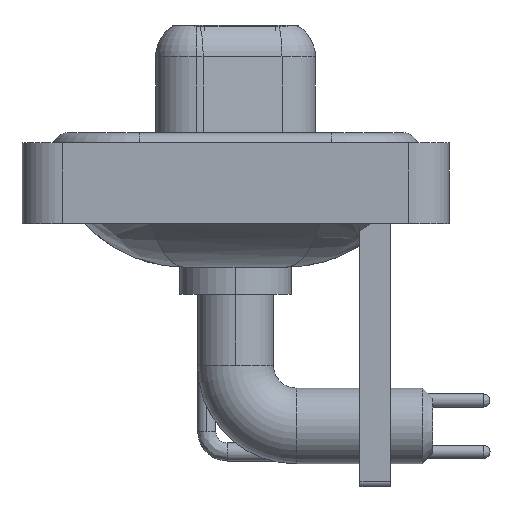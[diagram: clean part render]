
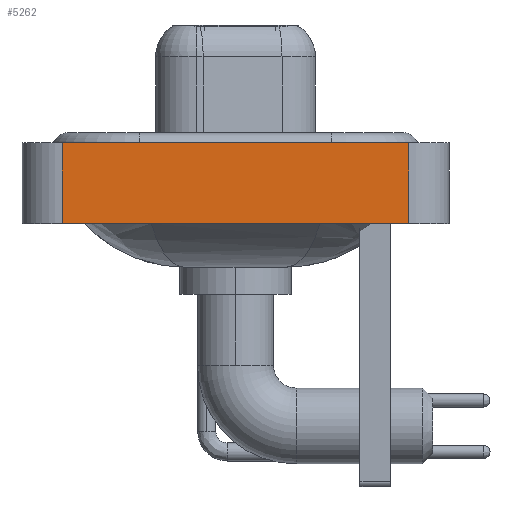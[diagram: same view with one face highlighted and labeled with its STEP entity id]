
A CAD part, left-side view. The second image highlights one B-rep face of the part: STEP entity #5262.
In plain terms, the highlighted planar face has unit normal (-1, 0, 0).
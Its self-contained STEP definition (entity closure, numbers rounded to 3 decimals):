
#1108 = VECTOR ( 'NONE', #15501, 1000. ) ;
#1297 = EDGE_CURVE ( 'NONE', #2075, #3065, #6027, .T. ) ;
#1966 = DIRECTION ( 'NONE',  ( 0., -1., 0. ) ) ;
#2075 = VERTEX_POINT ( 'NONE', #19175 ) ;
#2217 = CARTESIAN_POINT ( 'NONE',  ( -7.35, -8.55, -3.6 ) ) ;
#2495 = ORIENTED_EDGE ( 'NONE', *, *, #7056, .F. ) ;
#3065 = VERTEX_POINT ( 'NONE', #19233 ) ;
#3313 = PLANE ( 'NONE',  #6069 ) ;
#4199 = VECTOR ( 'NONE', #4363, 1000. ) ;
#4363 = DIRECTION ( 'NONE',  ( 0., -1., 0. ) ) ;
#4725 = FACE_OUTER_BOUND ( 'NONE', #13843, .T. ) ;
#5262 = ADVANCED_FACE ( 'NONE', ( #4725 ), #3313, .T. ) ;
#5466 = LINE ( 'NONE', #13095, #1108 ) ;
#6027 = LINE ( 'NONE', #10835, #11275 ) ;
#6069 = AXIS2_PLACEMENT_3D ( 'NONE', #14929, #8997, #11221 ) ;
#6114 = ORIENTED_EDGE ( 'NONE', *, *, #1297, .F. ) ;
#7056 = EDGE_CURVE ( 'NONE', #3065, #20073, #16213, .T. ) ;
#8377 = CARTESIAN_POINT ( 'NONE',  ( -7.35, -8.55, 0.4 ) ) ;
#8997 = DIRECTION ( 'NONE',  ( -1., 0., 0. ) ) ;
#9593 = EDGE_CURVE ( 'NONE', #24338, #20073, #5466, .T. ) ;
#10804 = ORIENTED_EDGE ( 'NONE', *, *, #23355, .T. ) ;
#10835 = CARTESIAN_POINT ( 'NONE',  ( -7.35, 8.55, -3.6 ) ) ;
#10899 = ORIENTED_EDGE ( 'NONE', *, *, #9593, .T. ) ;
#11221 = DIRECTION ( 'NONE',  ( 0., 0., 1. ) ) ;
#11275 = VECTOR ( 'NONE', #12360, 1000. ) ;
#11338 = CARTESIAN_POINT ( 'NONE',  ( -7.35, -8.55, 0.4 ) ) ;
#11789 = LINE ( 'NONE', #2217, #22003 ) ;
#12360 = DIRECTION ( 'NONE',  ( 0., 0., 1. ) ) ;
#13095 = CARTESIAN_POINT ( 'NONE',  ( -7.35, -8.55, -3.6 ) ) ;
#13843 = EDGE_LOOP ( 'NONE', ( #10899, #2495, #6114, #10804 ) ) ;
#14929 = CARTESIAN_POINT ( 'NONE',  ( -7.35, -8.55, -3.6 ) ) ;
#15501 = DIRECTION ( 'NONE',  ( 0., 0., 1. ) ) ;
#16213 = LINE ( 'NONE', #8377, #4199 ) ;
#19175 = CARTESIAN_POINT ( 'NONE',  ( -7.35, 8.55, -3.6 ) ) ;
#19233 = CARTESIAN_POINT ( 'NONE',  ( -7.35, 8.55, 0.4 ) ) ;
#20073 = VERTEX_POINT ( 'NONE', #11338 ) ;
#22003 = VECTOR ( 'NONE', #1966, 1000. ) ;
#23355 = EDGE_CURVE ( 'NONE', #2075, #24338, #11789, .T. ) ;
#23597 = CARTESIAN_POINT ( 'NONE',  ( -7.35, -8.55, -3.6 ) ) ;
#24338 = VERTEX_POINT ( 'NONE', #23597 ) ;
